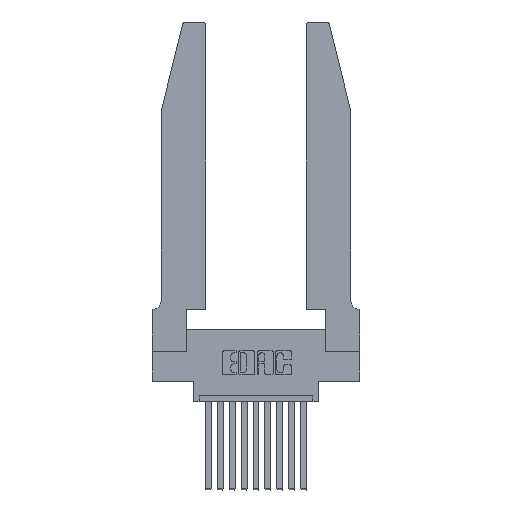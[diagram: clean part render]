
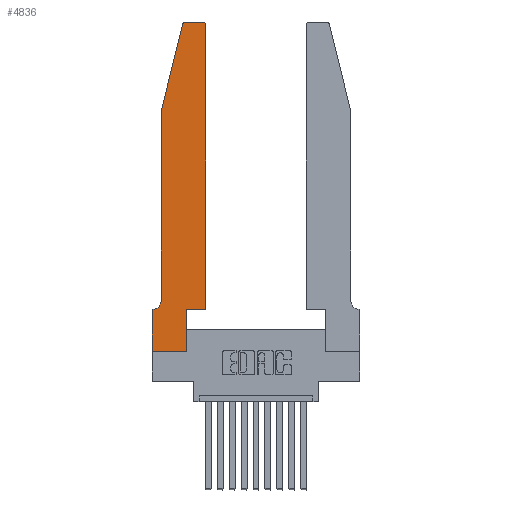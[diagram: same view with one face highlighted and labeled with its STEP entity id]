
A CAD part, top view. The second image highlights one B-rep face of the part: STEP entity #4836.
In plain terms, the highlighted planar face has unit normal (0, 0, 1).
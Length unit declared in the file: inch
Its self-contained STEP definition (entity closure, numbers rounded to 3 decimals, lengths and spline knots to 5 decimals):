
#140 = DIRECTION ( 'NONE',  ( 1., 0., 0. ) ) ;
#234 = EDGE_CURVE ( 'NONE', #5439, #6162, #14833, .T. ) ;
#346 = DIRECTION ( 'NONE',  ( 1., 0., 0. ) ) ;
#582 = CARTESIAN_POINT ( 'NONE',  ( 0., 0., 0.37 ) ) ;
#829 = CIRCLE ( 'NONE', #10734, 0.03 ) ;
#894 = ORIENTED_EDGE ( 'NONE', *, *, #14660, .T. ) ;
#965 = EDGE_LOOP ( 'NONE', ( #1853, #1914, #7272, #2496, #2190, #5614, #4542, #3714, #894, #12202, #11215, #11013 ) ) ;
#1180 = CARTESIAN_POINT ( 'NONE',  ( 0.0755, 0.42, 0.37 ) ) ;
#1397 = CARTESIAN_POINT ( 'NONE',  ( 0.2865, 0.35, 0.37 ) ) ;
#1427 = DIRECTION ( 'NONE',  ( 1., 0., 0. ) ) ;
#1596 = CARTESIAN_POINT ( 'NONE',  ( 0.284, 2.72, 0.37 ) ) ;
#1604 = CARTESIAN_POINT ( 'NONE',  ( 0.0755, 2., 0.37 ) ) ;
#1721 = DIRECTION ( 'NONE',  ( 0., -1., 0. ) ) ;
#1853 = ORIENTED_EDGE ( 'NONE', *, *, #2767, .T. ) ;
#1914 = ORIENTED_EDGE ( 'NONE', *, *, #14263, .T. ) ;
#2190 = ORIENTED_EDGE ( 'NONE', *, *, #10864, .T. ) ;
#2222 = VERTEX_POINT ( 'NONE', #10932 ) ;
#2496 = ORIENTED_EDGE ( 'NONE', *, *, #15938, .T. ) ;
#2767 = EDGE_CURVE ( 'NONE', #4575, #8250, #8255, .T. ) ;
#2888 = CARTESIAN_POINT ( 'NONE',  ( 0.4505, 2.72, 0.37 ) ) ;
#3189 = CARTESIAN_POINT ( 'NONE',  ( 0.0755, 2., 0.37 ) ) ;
#3527 = CARTESIAN_POINT ( 'NONE',  ( 0.0055, 0.42, 0.37 ) ) ;
#3714 = ORIENTED_EDGE ( 'NONE', *, *, #14624, .T. ) ;
#4175 = VERTEX_POINT ( 'NONE', #9988 ) ;
#4425 = CARTESIAN_POINT ( 'NONE',  ( 0., 0.35, 0.37 ) ) ;
#4542 = ORIENTED_EDGE ( 'NONE', *, *, #13742, .T. ) ;
#4575 = VERTEX_POINT ( 'NONE', #14102 ) ;
#4640 = CIRCLE ( 'NONE', #15669, 0.03 ) ;
#4752 = DIRECTION ( 'NONE',  ( -1., 0., 0. ) ) ;
#4765 = DIRECTION ( 'NONE',  ( -1., 0., 0. ) ) ;
#4822 = CARTESIAN_POINT ( 'NONE',  ( 0.4505, 0.35, 0.37 ) ) ;
#4836 = ADVANCED_FACE ( 'NONE', ( #15845 ), #6132, .T. ) ;
#4933 = DIRECTION ( 'NONE',  ( 1., 0., 0. ) ) ;
#4994 = LINE ( 'NONE', #8583, #13101 ) ;
#5102 = AXIS2_PLACEMENT_3D ( 'NONE', #7518, #15877, #4933 ) ;
#5159 = CARTESIAN_POINT ( 'NONE',  ( 0.0055, 0.35, 0.37 ) ) ;
#5439 = VERTEX_POINT ( 'NONE', #7349 ) ;
#5614 = ORIENTED_EDGE ( 'NONE', *, *, #14596, .T. ) ;
#5723 = EDGE_CURVE ( 'NONE', #6162, #4575, #829, .T. ) ;
#5934 = LINE ( 'NONE', #12999, #12058 ) ;
#6132 = PLANE ( 'NONE',  #5102 ) ;
#6156 = DIRECTION ( 'NONE',  ( 1., 0., 0. ) ) ;
#6162 = VERTEX_POINT ( 'NONE', #2888 ) ;
#6987 = VECTOR ( 'NONE', #1721, 39.37008 ) ;
#7272 = ORIENTED_EDGE ( 'NONE', *, *, #9784, .T. ) ;
#7349 = CARTESIAN_POINT ( 'NONE',  ( 0.4505, 0.35, 0.37 ) ) ;
#7364 = LINE ( 'NONE', #582, #6987 ) ;
#7515 = VERTEX_POINT ( 'NONE', #12036 ) ;
#7518 = CARTESIAN_POINT ( 'NONE',  ( 0., 0.35, 0.37 ) ) ;
#7893 = LINE ( 'NONE', #1397, #11904 ) ;
#8250 = VERTEX_POINT ( 'NONE', #15727 ) ;
#8255 = LINE ( 'NONE', #13038, #14789 ) ;
#8541 = EDGE_CURVE ( 'NONE', #4175, #5439, #11525, .T. ) ;
#8583 = CARTESIAN_POINT ( 'NONE',  ( 0.0755, 0.35, 0.37 ) ) ;
#8640 = VERTEX_POINT ( 'NONE', #1604 ) ;
#8846 = DIRECTION ( 'NONE',  ( 0., 1., 0. ) ) ;
#8847 = VECTOR ( 'NONE', #12940, 39.37008 ) ;
#8878 = CARTESIAN_POINT ( 'NONE',  ( 0.4205, 2.72, 0.37 ) ) ;
#9270 = DIRECTION ( 'NONE',  ( 0., -1., 0. ) ) ;
#9406 = CARTESIAN_POINT ( 'NONE',  ( 0.4505, 0.35, 0.37 ) ) ;
#9522 = VERTEX_POINT ( 'NONE', #13746 ) ;
#9574 = CARTESIAN_POINT ( 'NONE',  ( 0., 0., 0.37 ) ) ;
#9784 = EDGE_CURVE ( 'NONE', #2222, #8640, #14620, .T. ) ;
#9978 = LINE ( 'NONE', #9574, #11134 ) ;
#9988 = CARTESIAN_POINT ( 'NONE',  ( 0.2865, 0.35, 0.37 ) ) ;
#10532 = DIRECTION ( 'NONE',  ( 0., 1., 0. ) ) ;
#10559 = VERTEX_POINT ( 'NONE', #5159 ) ;
#10734 = AXIS2_PLACEMENT_3D ( 'NONE', #8878, #14980, #1427 ) ;
#10864 = EDGE_CURVE ( 'NONE', #14602, #10559, #11292, .T. ) ;
#10932 = CARTESIAN_POINT ( 'NONE',  ( 0.25487, 2.72718, 0.37 ) ) ;
#11013 = ORIENTED_EDGE ( 'NONE', *, *, #5723, .T. ) ;
#11134 = VECTOR ( 'NONE', #6156, 39.37008 ) ;
#11215 = ORIENTED_EDGE ( 'NONE', *, *, #234, .T. ) ;
#11249 = DIRECTION ( 'NONE',  ( 0., 0., 1. ) ) ;
#11292 = CIRCLE ( 'NONE', #11354, 0.07 ) ;
#11354 = AXIS2_PLACEMENT_3D ( 'NONE', #3527, #12113, #4765 ) ;
#11525 = LINE ( 'NONE', #4822, #14254 ) ;
#11550 = VECTOR ( 'NONE', #10532, 39.37008 ) ;
#11904 = VECTOR ( 'NONE', #8846, 39.37008 ) ;
#12036 = CARTESIAN_POINT ( 'NONE',  ( 0., 0., 0.37 ) ) ;
#12058 = VECTOR ( 'NONE', #9270, 39.37008 ) ;
#12073 = DIRECTION ( 'NONE',  ( -1., 0., 0. ) ) ;
#12113 = DIRECTION ( 'NONE',  ( 0., 0., -1. ) ) ;
#12202 = ORIENTED_EDGE ( 'NONE', *, *, #8541, .T. ) ;
#12940 = DIRECTION ( 'NONE',  ( -0.239, -0.971, 0. ) ) ;
#12999 = CARTESIAN_POINT ( 'NONE',  ( 0.0755, 2., 0.37 ) ) ;
#13038 = CARTESIAN_POINT ( 'NONE',  ( 0.2605, 2.75, 0.37 ) ) ;
#13101 = VECTOR ( 'NONE', #4752, 39.37008 ) ;
#13742 = EDGE_CURVE ( 'NONE', #15544, #7515, #7364, .T. ) ;
#13746 = CARTESIAN_POINT ( 'NONE',  ( 0.2865, 0., 0.37 ) ) ;
#14102 = CARTESIAN_POINT ( 'NONE',  ( 0.4205, 2.75, 0.37 ) ) ;
#14254 = VECTOR ( 'NONE', #140, 39.37008 ) ;
#14263 = EDGE_CURVE ( 'NONE', #8250, #2222, #4640, .T. ) ;
#14596 = EDGE_CURVE ( 'NONE', #10559, #15544, #4994, .T. ) ;
#14602 = VERTEX_POINT ( 'NONE', #1180 ) ;
#14620 = LINE ( 'NONE', #3189, #8847 ) ;
#14624 = EDGE_CURVE ( 'NONE', #7515, #9522, #9978, .T. ) ;
#14660 = EDGE_CURVE ( 'NONE', #9522, #4175, #7893, .T. ) ;
#14789 = VECTOR ( 'NONE', #12073, 39.37008 ) ;
#14833 = LINE ( 'NONE', #9406, #11550 ) ;
#14980 = DIRECTION ( 'NONE',  ( 0., 0., 1. ) ) ;
#15544 = VERTEX_POINT ( 'NONE', #4425 ) ;
#15669 = AXIS2_PLACEMENT_3D ( 'NONE', #1596, #11249, #346 ) ;
#15727 = CARTESIAN_POINT ( 'NONE',  ( 0.284, 2.75, 0.37 ) ) ;
#15845 = FACE_OUTER_BOUND ( 'NONE', #965, .T. ) ;
#15877 = DIRECTION ( 'NONE',  ( 0., 0., 1. ) ) ;
#15938 = EDGE_CURVE ( 'NONE', #8640, #14602, #5934, .T. ) ;
